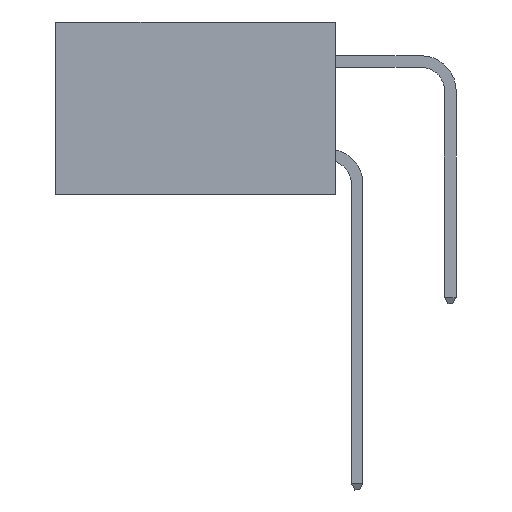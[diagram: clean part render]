
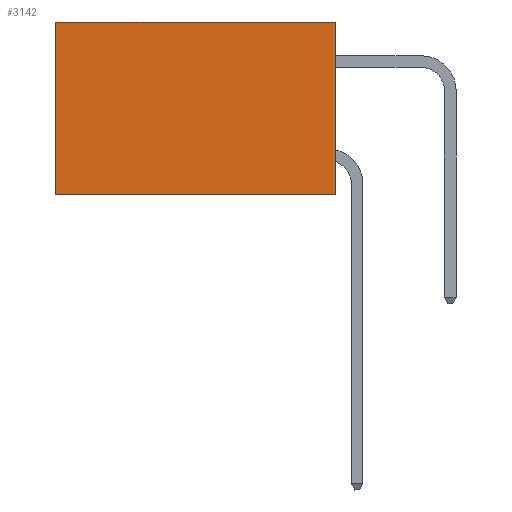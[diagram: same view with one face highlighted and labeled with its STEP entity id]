
A CAD part, left-side view. The second image highlights one B-rep face of the part: STEP entity #3142.
In plain terms, the highlighted planar face has unit normal (-1, 0, 0).
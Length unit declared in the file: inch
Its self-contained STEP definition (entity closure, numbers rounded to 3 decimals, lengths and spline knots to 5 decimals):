
#462 = VECTOR ( 'NONE', #1857, 39.37008 ) ;
#658 = EDGE_CURVE ( 'NONE', #11203, #9533, #15314, .T. ) ;
#1035 = VECTOR ( 'NONE', #11007, 39.37008 ) ;
#1857 = DIRECTION ( 'NONE',  ( 0., 0., -1. ) ) ;
#2215 = EDGE_CURVE ( 'NONE', #23192, #11203, #14267, .T. ) ;
#2415 = EDGE_CURVE ( 'NONE', #23192, #11228, #26063, .T. ) ;
#2436 = ORIENTED_EDGE ( 'NONE', *, *, #3397, .F. ) ;
#3086 = VECTOR ( 'NONE', #3422, 39.37008 ) ;
#3142 = ADVANCED_FACE ( 'NONE', ( #25380 ), #16502, .F. ) ;
#3254 = ORIENTED_EDGE ( 'NONE', *, *, #2215, .T. ) ;
#3397 = EDGE_CURVE ( 'NONE', #11228, #9533, #24042, .T. ) ;
#3422 = DIRECTION ( 'NONE',  ( 0., 1., 0. ) ) ;
#3783 = AXIS2_PLACEMENT_3D ( 'NONE', #6322, #4127, #10365 ) ;
#4127 = DIRECTION ( 'NONE',  ( 1., 0., 0. ) ) ;
#4596 = CARTESIAN_POINT ( 'NONE',  ( 0.2875, 0.6, -0.37 ) ) ;
#4681 = CARTESIAN_POINT ( 'NONE',  ( 0.2875, 0., -0.37 ) ) ;
#6122 = VECTOR ( 'NONE', #16526, 39.37008 ) ;
#6322 = CARTESIAN_POINT ( 'NONE',  ( 0.2875, 0., 0. ) ) ;
#7981 = CARTESIAN_POINT ( 'NONE',  ( 0.2875, 0.6, 0. ) ) ;
#8850 = ORIENTED_EDGE ( 'NONE', *, *, #2415, .F. ) ;
#9533 = VERTEX_POINT ( 'NONE', #4596 ) ;
#10365 = DIRECTION ( 'NONE',  ( 0., 0., -1. ) ) ;
#11007 = DIRECTION ( 'NONE',  ( 0., 1., 0. ) ) ;
#11203 = VERTEX_POINT ( 'NONE', #22233 ) ;
#11228 = VERTEX_POINT ( 'NONE', #24267 ) ;
#13908 = EDGE_LOOP ( 'NONE', ( #19507, #2436, #8850, #3254 ) ) ;
#14267 = LINE ( 'NONE', #23825, #3086 ) ;
#14444 = CARTESIAN_POINT ( 'NONE',  ( 0.2875, 0., 0. ) ) ;
#15314 = LINE ( 'NONE', #7981, #6122 ) ;
#16502 = PLANE ( 'NONE',  #3783 ) ;
#16526 = DIRECTION ( 'NONE',  ( 0., 0., -1. ) ) ;
#17414 = CARTESIAN_POINT ( 'NONE',  ( 0.2875, 0., 0. ) ) ;
#19507 = ORIENTED_EDGE ( 'NONE', *, *, #658, .T. ) ;
#22233 = CARTESIAN_POINT ( 'NONE',  ( 0.2875, 0.6, 0. ) ) ;
#23192 = VERTEX_POINT ( 'NONE', #17414 ) ;
#23825 = CARTESIAN_POINT ( 'NONE',  ( 0.2875, 0., 0. ) ) ;
#24042 = LINE ( 'NONE', #4681, #1035 ) ;
#24267 = CARTESIAN_POINT ( 'NONE',  ( 0.2875, 0., -0.37 ) ) ;
#25380 = FACE_OUTER_BOUND ( 'NONE', #13908, .T. ) ;
#26063 = LINE ( 'NONE', #14444, #462 ) ;
